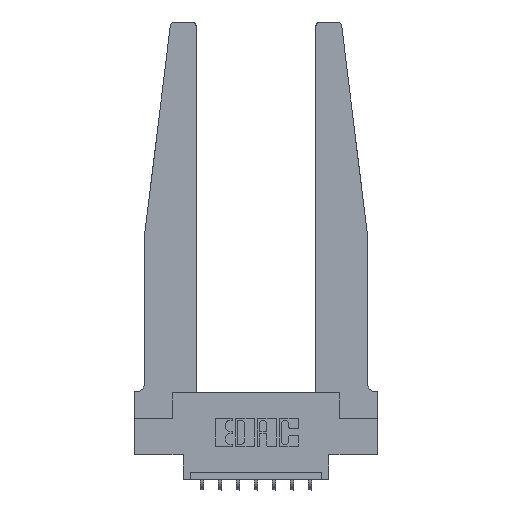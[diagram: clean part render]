
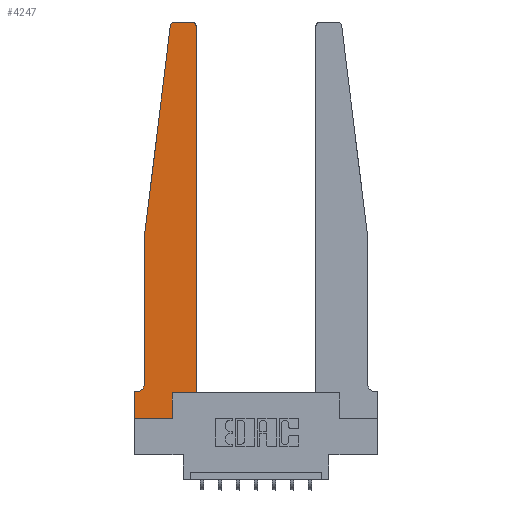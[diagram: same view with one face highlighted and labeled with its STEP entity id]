
A CAD part, top view. The second image highlights one B-rep face of the part: STEP entity #4247.
In plain terms, the highlighted planar face has unit normal (0, 0, 1).
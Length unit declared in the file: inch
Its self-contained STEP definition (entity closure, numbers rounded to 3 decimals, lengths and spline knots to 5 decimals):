
#23 = EDGE_CURVE ( 'NONE', #12661, #12935, #181, .T. ) ;
#163 = CARTESIAN_POINT ( 'NONE',  ( 0.425, 0.18, 0.37 ) ) ;
#181 = LINE ( 'NONE', #12561, #11084 ) ;
#516 = EDGE_CURVE ( 'NONE', #12935, #13785, #9398, .T. ) ;
#932 = DIRECTION ( 'NONE',  ( 1., 0., 0. ) ) ;
#937 = EDGE_CURVE ( 'NONE', #5168, #4911, #8828, .T. ) ;
#1136 = ORIENTED_EDGE ( 'NONE', *, *, #11311, .T. ) ;
#1339 = CARTESIAN_POINT ( 'NONE',  ( 0.065, 1.25, 0.37 ) ) ;
#1604 = CARTESIAN_POINT ( 'NONE',  ( 0.065, 1.25, 0.37 ) ) ;
#1726 = VECTOR ( 'NONE', #10273, 39.37008 ) ;
#1800 = DIRECTION ( 'NONE',  ( 0., 0., 1. ) ) ;
#1882 = CIRCLE ( 'NONE', #5146, 0.03 ) ;
#2446 = CARTESIAN_POINT ( 'NONE',  ( 0.425, 0.18, 0.37 ) ) ;
#2512 = VECTOR ( 'NONE', #2745, 39.37008 ) ;
#2578 = DIRECTION ( 'NONE',  ( -1., 0., 0. ) ) ;
#2652 = VECTOR ( 'NONE', #10411, 39.37008 ) ;
#2745 = DIRECTION ( 'NONE',  ( 0., 1., 0. ) ) ;
#2897 = DIRECTION ( 'NONE',  ( 1., 0., 0. ) ) ;
#3046 = ORIENTED_EDGE ( 'NONE', *, *, #937, .T. ) ;
#3593 = DIRECTION ( 'NONE',  ( 1., 0., 0. ) ) ;
#3663 = EDGE_CURVE ( 'NONE', #4911, #5714, #8613, .T. ) ;
#3877 = ORIENTED_EDGE ( 'NONE', *, *, #5919, .T. ) ;
#4020 = DIRECTION ( 'NONE',  ( -1., 0., 0. ) ) ;
#4124 = ORIENTED_EDGE ( 'NONE', *, *, #23, .T. ) ;
#4179 = VECTOR ( 'NONE', #7230, 39.37008 ) ;
#4247 = ADVANCED_FACE ( 'NONE', ( #13650 ), #6660, .T. ) ;
#4278 = CIRCLE ( 'NONE', #8007, 0.03 ) ;
#4393 = LINE ( 'NONE', #1339, #1726 ) ;
#4403 = CARTESIAN_POINT ( 'NONE',  ( 0.065, 0.2375, 0.37 ) ) ;
#4441 = VERTEX_POINT ( 'NONE', #8705 ) ;
#4775 = CARTESIAN_POINT ( 'NONE',  ( 0.2605, 0.18, 0.37 ) ) ;
#4911 = VERTEX_POINT ( 'NONE', #6463 ) ;
#5146 = AXIS2_PLACEMENT_3D ( 'NONE', #8199, #12711, #8275 ) ;
#5168 = VERTEX_POINT ( 'NONE', #4403 ) ;
#5208 = CARTESIAN_POINT ( 'NONE',  ( 0., 0., 0.37 ) ) ;
#5232 = ORIENTED_EDGE ( 'NONE', *, *, #13451, .T. ) ;
#5293 = EDGE_LOOP ( 'NONE', ( #7335, #6903, #1136, #12395, #3046, #10408, #3877, #4124, #11996, #5232, #7199, #7211 ) ) ;
#5700 = CARTESIAN_POINT ( 'NONE',  ( 0.065, 1.25, 0.37 ) ) ;
#5714 = VERTEX_POINT ( 'NONE', #11088 ) ;
#5752 = DIRECTION ( 'NONE',  ( 0., 1., 0. ) ) ;
#5834 = CARTESIAN_POINT ( 'NONE',  ( 0., 0., 0.37 ) ) ;
#5904 = CARTESIAN_POINT ( 'NONE',  ( 0.25, 2.75, 0.37 ) ) ;
#5919 = EDGE_CURVE ( 'NONE', #5714, #12661, #8176, .T. ) ;
#6389 = CARTESIAN_POINT ( 'NONE',  ( 0.425, 0.18, 0.37 ) ) ;
#6463 = CARTESIAN_POINT ( 'NONE',  ( 0.015, 0.1875, 0.37 ) ) ;
#6660 = PLANE ( 'NONE',  #8147 ) ;
#6741 = CARTESIAN_POINT ( 'NONE',  ( 0.27653, 2.75, 0.37 ) ) ;
#6896 = EDGE_CURVE ( 'NONE', #10606, #14343, #1882, .T. ) ;
#6903 = ORIENTED_EDGE ( 'NONE', *, *, #6896, .T. ) ;
#7034 = CARTESIAN_POINT ( 'NONE',  ( 0.2605, 0.18, 0.37 ) ) ;
#7199 = ORIENTED_EDGE ( 'NONE', *, *, #7464, .T. ) ;
#7211 = ORIENTED_EDGE ( 'NONE', *, *, #12669, .T. ) ;
#7230 = DIRECTION ( 'NONE',  ( 0., -1., 0. ) ) ;
#7335 = ORIENTED_EDGE ( 'NONE', *, *, #10034, .T. ) ;
#7464 = EDGE_CURVE ( 'NONE', #14157, #4441, #11365, .T. ) ;
#8007 = AXIS2_PLACEMENT_3D ( 'NONE', #13961, #1800, #2897 ) ;
#8039 = DIRECTION ( 'NONE',  ( 1., 0., 0. ) ) ;
#8107 = DIRECTION ( 'NONE',  ( 0., 0., -1. ) ) ;
#8147 = AXIS2_PLACEMENT_3D ( 'NONE', #11175, #12429, #3593 ) ;
#8176 = LINE ( 'NONE', #5834, #4179 ) ;
#8199 = CARTESIAN_POINT ( 'NONE',  ( 0.27653, 2.72, 0.37 ) ) ;
#8275 = DIRECTION ( 'NONE',  ( 1., 0., 0. ) ) ;
#8494 = VERTEX_POINT ( 'NONE', #9750 ) ;
#8613 = LINE ( 'NONE', #14071, #10405 ) ;
#8705 = CARTESIAN_POINT ( 'NONE',  ( 0.425, 2.72, 0.37 ) ) ;
#8828 = CIRCLE ( 'NONE', #9553, 0.05 ) ;
#9154 = CARTESIAN_POINT ( 'NONE',  ( 0.2605, 0., 0.37 ) ) ;
#9398 = LINE ( 'NONE', #4775, #2512 ) ;
#9553 = AXIS2_PLACEMENT_3D ( 'NONE', #13712, #8107, #2578 ) ;
#9609 = VECTOR ( 'NONE', #5752, 39.37008 ) ;
#9750 = CARTESIAN_POINT ( 'NONE',  ( 0.395, 2.75, 0.37 ) ) ;
#10034 = EDGE_CURVE ( 'NONE', #8494, #10606, #11520, .T. ) ;
#10255 = LINE ( 'NONE', #1604, #11570 ) ;
#10273 = DIRECTION ( 'NONE',  ( 0., -1., 0. ) ) ;
#10405 = VECTOR ( 'NONE', #4020, 39.37008 ) ;
#10408 = ORIENTED_EDGE ( 'NONE', *, *, #3663, .T. ) ;
#10411 = DIRECTION ( 'NONE',  ( -1., 0., 0. ) ) ;
#10606 = VERTEX_POINT ( 'NONE', #6741 ) ;
#10916 = EDGE_CURVE ( 'NONE', #14109, #5168, #4393, .T. ) ;
#11084 = VECTOR ( 'NONE', #8039, 39.37008 ) ;
#11088 = CARTESIAN_POINT ( 'NONE',  ( 0., 0.1875, 0.37 ) ) ;
#11175 = CARTESIAN_POINT ( 'NONE',  ( 0., 0.1875, 0.37 ) ) ;
#11311 = EDGE_CURVE ( 'NONE', #14343, #14109, #10255, .T. ) ;
#11365 = LINE ( 'NONE', #163, #9609 ) ;
#11520 = LINE ( 'NONE', #5904, #2652 ) ;
#11570 = VECTOR ( 'NONE', #11657, 39.37008 ) ;
#11657 = DIRECTION ( 'NONE',  ( -0.122, -0.992, 0. ) ) ;
#11965 = CARTESIAN_POINT ( 'NONE',  ( 0.24675, 2.72367, 0.37 ) ) ;
#11996 = ORIENTED_EDGE ( 'NONE', *, *, #516, .T. ) ;
#12395 = ORIENTED_EDGE ( 'NONE', *, *, #10916, .T. ) ;
#12429 = DIRECTION ( 'NONE',  ( 0., 0., 1. ) ) ;
#12561 = CARTESIAN_POINT ( 'NONE',  ( 0., 0., 0.37 ) ) ;
#12661 = VERTEX_POINT ( 'NONE', #5208 ) ;
#12669 = EDGE_CURVE ( 'NONE', #4441, #8494, #4278, .T. ) ;
#12711 = DIRECTION ( 'NONE',  ( 0., 0., 1. ) ) ;
#12935 = VERTEX_POINT ( 'NONE', #9154 ) ;
#12965 = LINE ( 'NONE', #6389, #14142 ) ;
#13451 = EDGE_CURVE ( 'NONE', #13785, #14157, #12965, .T. ) ;
#13650 = FACE_OUTER_BOUND ( 'NONE', #5293, .T. ) ;
#13712 = CARTESIAN_POINT ( 'NONE',  ( 0.015, 0.2375, 0.37 ) ) ;
#13785 = VERTEX_POINT ( 'NONE', #7034 ) ;
#13961 = CARTESIAN_POINT ( 'NONE',  ( 0.395, 2.72, 0.37 ) ) ;
#14071 = CARTESIAN_POINT ( 'NONE',  ( 0.065, 0.1875, 0.37 ) ) ;
#14109 = VERTEX_POINT ( 'NONE', #5700 ) ;
#14142 = VECTOR ( 'NONE', #932, 39.37008 ) ;
#14157 = VERTEX_POINT ( 'NONE', #2446 ) ;
#14343 = VERTEX_POINT ( 'NONE', #11965 ) ;
